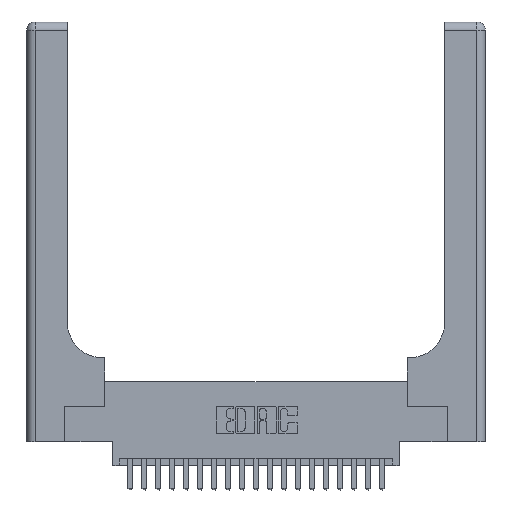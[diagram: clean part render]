
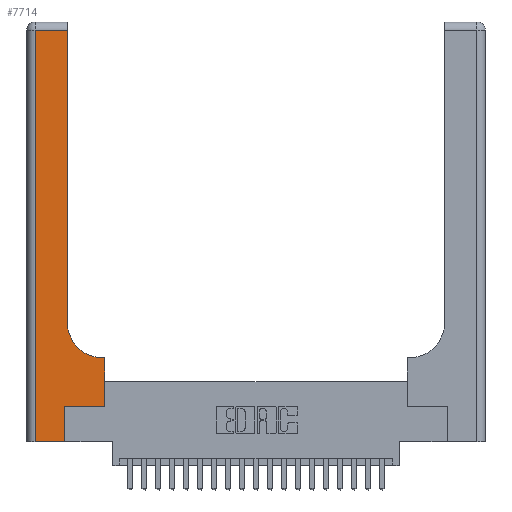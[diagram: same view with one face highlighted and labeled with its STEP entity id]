
A CAD part, top view. The second image highlights one B-rep face of the part: STEP entity #7714.
In plain terms, the highlighted planar face has unit normal (0, 0, 1).
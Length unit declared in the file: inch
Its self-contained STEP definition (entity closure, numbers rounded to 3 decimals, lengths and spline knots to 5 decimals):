
#995 = DIRECTION ( 'NONE',  ( 1., 0., 0. ) ) ;
#1264 = EDGE_CURVE ( 'NONE', #13148, #18870, #8707, .T. ) ;
#1267 = DIRECTION ( 'NONE',  ( 0., 0., -1. ) ) ;
#1287 = DIRECTION ( 'NONE',  ( 1., 0., 0. ) ) ;
#1311 = DIRECTION ( 'NONE',  ( 0., 0., -1. ) ) ;
#1331 = CARTESIAN_POINT ( 'NONE',  ( 0.5415, 0.85, 0.37 ) ) ;
#1995 = VERTEX_POINT ( 'NONE', #3408 ) ;
#2083 = LINE ( 'NONE', #6548, #20828 ) ;
#2643 = CARTESIAN_POINT ( 'NONE',  ( 0.2915, 0.85, 0.37 ) ) ;
#2907 = EDGE_CURVE ( 'NONE', #14473, #1995, #22799, .T. ) ;
#3077 = ORIENTED_EDGE ( 'NONE', *, *, #22615, .T. ) ;
#3206 = ORIENTED_EDGE ( 'NONE', *, *, #18992, .T. ) ;
#3254 = LINE ( 'NONE', #19582, #17226 ) ;
#3408 = CARTESIAN_POINT ( 'NONE',  ( 0.5585, 0.6, 0.37 ) ) ;
#3794 = EDGE_CURVE ( 'NONE', #17511, #21073, #10928, .T. ) ;
#3958 = FACE_OUTER_BOUND ( 'NONE', #18332, .T. ) ;
#3962 = EDGE_CURVE ( 'NONE', #21073, #23200, #2083, .T. ) ;
#4234 = CARTESIAN_POINT ( 'NONE',  ( 0.5585, 0.25, 0.37 ) ) ;
#4366 = CARTESIAN_POINT ( 'NONE',  ( 0.5585, 0.25, 0.37 ) ) ;
#5508 = LINE ( 'NONE', #11604, #15233 ) ;
#5918 = LINE ( 'NONE', #11401, #15047 ) ;
#6003 = ORIENTED_EDGE ( 'NONE', *, *, #3962, .T. ) ;
#6548 = CARTESIAN_POINT ( 'NONE',  ( 0.06, 3., 0.37 ) ) ;
#6550 = CARTESIAN_POINT ( 'NONE',  ( 0.269, 0., 0.37 ) ) ;
#6558 = CARTESIAN_POINT ( 'NONE',  ( 0.2915, 3., 0.37 ) ) ;
#7714 = ADVANCED_FACE ( 'NONE', ( #3958 ), #21181, .F. ) ;
#7898 = DIRECTION ( 'NONE',  ( -1., 0., 0. ) ) ;
#7955 = DIRECTION ( 'NONE',  ( 0., 1., 0. ) ) ;
#8131 = VERTEX_POINT ( 'NONE', #14801 ) ;
#8414 = DIRECTION ( 'NONE',  ( 0., 1., 0. ) ) ;
#8674 = CARTESIAN_POINT ( 'NONE',  ( 0.5415, 0.6, 0.37 ) ) ;
#8707 = CIRCLE ( 'NONE', #10936, 0.25 ) ;
#9211 = ORIENTED_EDGE ( 'NONE', *, *, #2907, .T. ) ;
#9633 = DIRECTION ( 'NONE',  ( -1., 0., 0. ) ) ;
#10262 = AXIS2_PLACEMENT_3D ( 'NONE', #12179, #1267, #14004 ) ;
#10756 = ORIENTED_EDGE ( 'NONE', *, *, #1264, .T. ) ;
#10928 = LINE ( 'NONE', #22314, #19406 ) ;
#10936 = AXIS2_PLACEMENT_3D ( 'NONE', #1331, #1311, #1287 ) ;
#11401 = CARTESIAN_POINT ( 'NONE',  ( 0.269, 0., 0.37 ) ) ;
#11604 = CARTESIAN_POINT ( 'NONE',  ( 0.2915, 0.6, 0.37 ) ) ;
#11993 = EDGE_CURVE ( 'NONE', #8131, #14473, #3254, .T. ) ;
#12179 = CARTESIAN_POINT ( 'NONE',  ( 0., 3., 0.37 ) ) ;
#12271 = ORIENTED_EDGE ( 'NONE', *, *, #3794, .T. ) ;
#12341 = EDGE_CURVE ( 'NONE', #1995, #13148, #5508, .T. ) ;
#13148 = VERTEX_POINT ( 'NONE', #8674 ) ;
#13226 = DIRECTION ( 'NONE',  ( 0., 1., 0. ) ) ;
#13729 = CARTESIAN_POINT ( 'NONE',  ( 0., 0., 0.37 ) ) ;
#13980 = CARTESIAN_POINT ( 'NONE',  ( 0.06, 2.94, 0.37 ) ) ;
#14004 = DIRECTION ( 'NONE',  ( -1., 0., 0. ) ) ;
#14449 = LINE ( 'NONE', #6558, #23453 ) ;
#14473 = VERTEX_POINT ( 'NONE', #4234 ) ;
#14545 = CARTESIAN_POINT ( 'NONE',  ( 0.2915, 2.94, 0.37 ) ) ;
#14801 = CARTESIAN_POINT ( 'NONE',  ( 0.269, 0.25, 0.37 ) ) ;
#14931 = CARTESIAN_POINT ( 'NONE',  ( 0.06, 0., 0.37 ) ) ;
#15047 = VECTOR ( 'NONE', #13226, 39.37008 ) ;
#15233 = VECTOR ( 'NONE', #7898, 39.37008 ) ;
#15906 = ORIENTED_EDGE ( 'NONE', *, *, #11993, .T. ) ;
#16461 = ORIENTED_EDGE ( 'NONE', *, *, #21545, .T. ) ;
#17226 = VECTOR ( 'NONE', #21403, 39.37008 ) ;
#17469 = DIRECTION ( 'NONE',  ( 0., -1., 0. ) ) ;
#17511 = VERTEX_POINT ( 'NONE', #14545 ) ;
#18204 = ORIENTED_EDGE ( 'NONE', *, *, #12341, .T. ) ;
#18332 = EDGE_LOOP ( 'NONE', ( #3206, #12271, #6003, #16461, #3077, #15906, #9211, #18204, #10756 ) ) ;
#18566 = VECTOR ( 'NONE', #7955, 39.37008 ) ;
#18870 = VERTEX_POINT ( 'NONE', #2643 ) ;
#18992 = EDGE_CURVE ( 'NONE', #18870, #17511, #14449, .T. ) ;
#19406 = VECTOR ( 'NONE', #9633, 39.37008 ) ;
#19582 = CARTESIAN_POINT ( 'NONE',  ( 0.269, 0.25, 0.37 ) ) ;
#20828 = VECTOR ( 'NONE', #17469, 39.37008 ) ;
#21073 = VERTEX_POINT ( 'NONE', #13980 ) ;
#21181 = PLANE ( 'NONE',  #10262 ) ;
#21403 = DIRECTION ( 'NONE',  ( 1., 0., 0. ) ) ;
#21545 = EDGE_CURVE ( 'NONE', #23200, #22789, #22180, .T. ) ;
#22180 = LINE ( 'NONE', #13729, #22733 ) ;
#22314 = CARTESIAN_POINT ( 'NONE',  ( 0., 2.94, 0.37 ) ) ;
#22615 = EDGE_CURVE ( 'NONE', #22789, #8131, #5918, .T. ) ;
#22733 = VECTOR ( 'NONE', #995, 39.37008 ) ;
#22789 = VERTEX_POINT ( 'NONE', #6550 ) ;
#22799 = LINE ( 'NONE', #4366, #18566 ) ;
#23200 = VERTEX_POINT ( 'NONE', #14931 ) ;
#23453 = VECTOR ( 'NONE', #8414, 39.37008 ) ;
